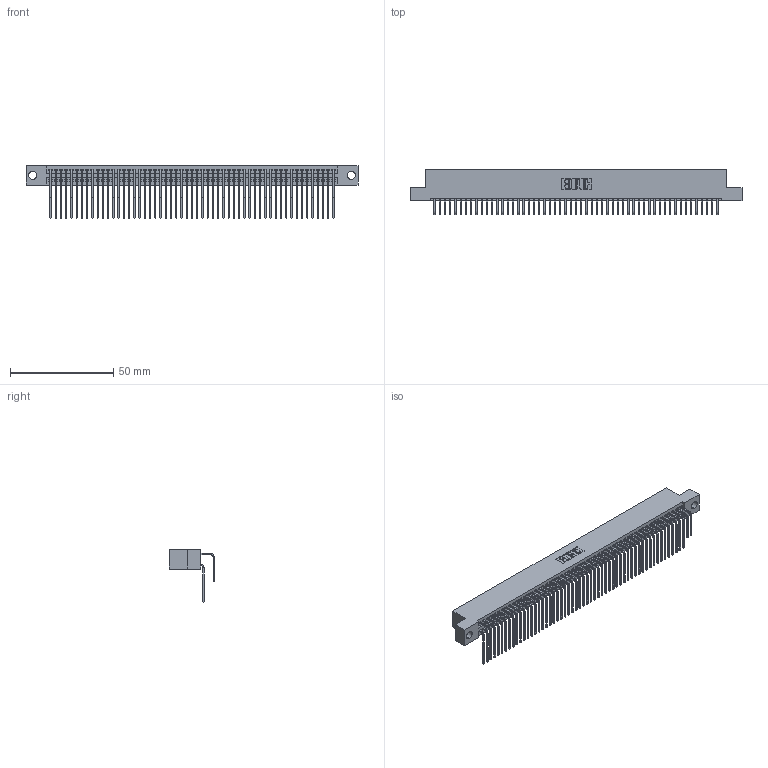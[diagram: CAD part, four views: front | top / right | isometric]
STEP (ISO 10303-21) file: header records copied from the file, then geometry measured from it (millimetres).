
FILE_DESCRIPTION (( 'STEP AP203' ), '1' );
FILE_NAME ('345-110-558-204.STEP', '2018-10-07T12:08:55', ( '' ), ( '' ), 'SwSTEP 2.0', 'SolidWorks 2016', '' );
FILE_SCHEMA (( 'CONFIG_CONTROL_DESIGN' ));
Length unit declared in the file: inch
Products named in the file (4): 345 Part_Flush Mounting Lugs - 0.156 Dia-TH; 345-110-558-204; 345-292-001_558 559 Tail - 1; 345-292-001_558 Tail - 2
Assembly tree (111 placements, depth 2):
  345-110-558-204
    345 Part_Flush Mounting Lugs - 0.156 Dia-TH
    345-292-001_558 559 Tail - 1  x55
    345-292-001_558 Tail - 2  x55
Bounding box: 160.91 x 21.83 x 25.53 mm (x, y, z)
Volume: 16298.2 mm3; surface area: 27142.4 mm2
Topology: 111 solids, 111 shells, 5846 faces, 17391 edges, 11446 vertices
Faces by surface type: plane 3930, cylinder 1916
Entity records: 43059 total; most frequent: CARTESIAN_POINT 7251, ORIENTED_EDGE 7134, DIRECTION 6351, EDGE_CURVE 3567, LINE 3175, VECTOR 3175, VERTEX_POINT 2374, AXIS2_PLACEMENT_3D 1588
